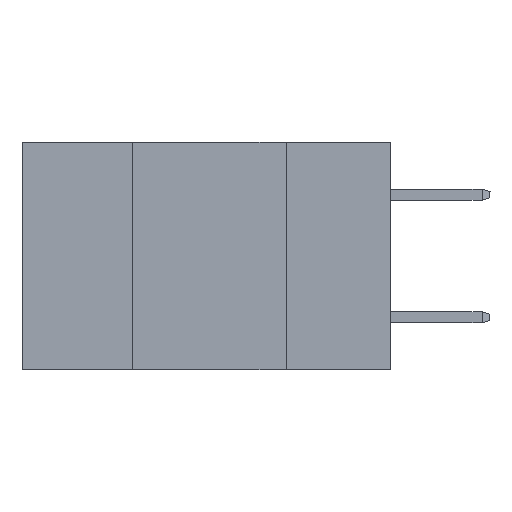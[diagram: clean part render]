
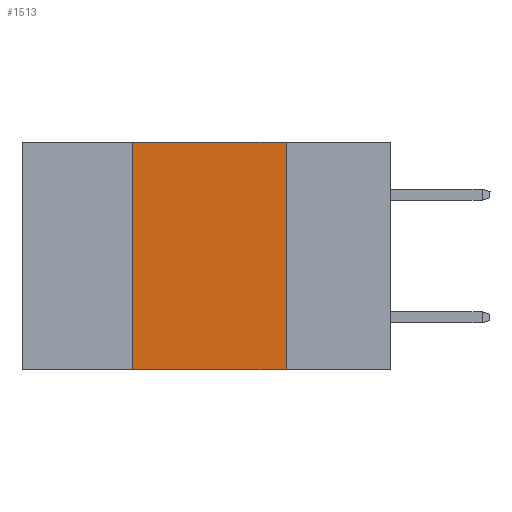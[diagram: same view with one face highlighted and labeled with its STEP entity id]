
A CAD part, left-side view. The second image highlights one B-rep face of the part: STEP entity #1513.
In plain terms, the highlighted planar face has unit normal (-1, 0, 0).
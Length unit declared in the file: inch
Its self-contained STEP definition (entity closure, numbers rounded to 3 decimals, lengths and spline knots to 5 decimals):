
#350 = DIRECTION ( 'NONE',  ( 0., -1., 0. ) ) ;
#381 = CARTESIAN_POINT ( 'NONE',  ( 0., 0.6, 0. ) ) ;
#929 = VECTOR ( 'NONE', #350, 39.37008 ) ;
#1307 = LINE ( 'NONE', #7881, #2280 ) ;
#1462 = DIRECTION ( 'NONE',  ( 0., 0., 1. ) ) ;
#1513 = ADVANCED_FACE ( 'NONE', ( #10741 ), #8039, .F. ) ;
#2052 = LINE ( 'NONE', #4029, #929 ) ;
#2280 = VECTOR ( 'NONE', #9779, 39.37008 ) ;
#2612 = CARTESIAN_POINT ( 'NONE',  ( 0., 0.42, 0. ) ) ;
#3262 = ORIENTED_EDGE ( 'NONE', *, *, #6087, .F. ) ;
#4029 = CARTESIAN_POINT ( 'NONE',  ( 0., 0.6, 0. ) ) ;
#4312 = LINE ( 'NONE', #2612, #10151 ) ;
#4717 = LINE ( 'NONE', #9422, #10984 ) ;
#5041 = VERTEX_POINT ( 'NONE', #7443 ) ;
#5862 = AXIS2_PLACEMENT_3D ( 'NONE', #381, #10855, #9824 ) ;
#6087 = EDGE_CURVE ( 'NONE', #9982, #8250, #2052, .T. ) ;
#6193 = ORIENTED_EDGE ( 'NONE', *, *, #8450, .F. ) ;
#6727 = CARTESIAN_POINT ( 'NONE',  ( 0., 0.42, -0.37 ) ) ;
#7124 = EDGE_LOOP ( 'NONE', ( #10554, #3262, #6193, #7618 ) ) ;
#7378 = CARTESIAN_POINT ( 'NONE',  ( 0., 0.17, 0. ) ) ;
#7443 = CARTESIAN_POINT ( 'NONE',  ( 0., 0.17, -0.37 ) ) ;
#7513 = DIRECTION ( 'NONE',  ( 0., 0., -1. ) ) ;
#7618 = ORIENTED_EDGE ( 'NONE', *, *, #7833, .T. ) ;
#7833 = EDGE_CURVE ( 'NONE', #9423, #5041, #1307, .T. ) ;
#7881 = CARTESIAN_POINT ( 'NONE',  ( 0., 0.6, -0.37 ) ) ;
#8039 = PLANE ( 'NONE',  #5862 ) ;
#8089 = CARTESIAN_POINT ( 'NONE',  ( 0., 0.42, 0. ) ) ;
#8250 = VERTEX_POINT ( 'NONE', #7378 ) ;
#8450 = EDGE_CURVE ( 'NONE', #9423, #9982, #4312, .T. ) ;
#9422 = CARTESIAN_POINT ( 'NONE',  ( 0., 0.17, 0. ) ) ;
#9423 = VERTEX_POINT ( 'NONE', #6727 ) ;
#9779 = DIRECTION ( 'NONE',  ( 0., -1., 0. ) ) ;
#9824 = DIRECTION ( 'NONE',  ( 0., 0., -1. ) ) ;
#9982 = VERTEX_POINT ( 'NONE', #8089 ) ;
#10151 = VECTOR ( 'NONE', #1462, 39.37008 ) ;
#10554 = ORIENTED_EDGE ( 'NONE', *, *, #11147, .F. ) ;
#10741 = FACE_OUTER_BOUND ( 'NONE', #7124, .T. ) ;
#10855 = DIRECTION ( 'NONE',  ( 1., 0., 0. ) ) ;
#10984 = VECTOR ( 'NONE', #7513, 39.37008 ) ;
#11147 = EDGE_CURVE ( 'NONE', #8250, #5041, #4717, .T. ) ;
